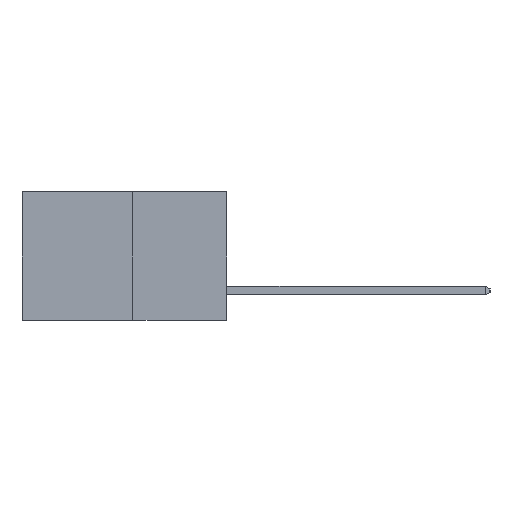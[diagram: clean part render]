
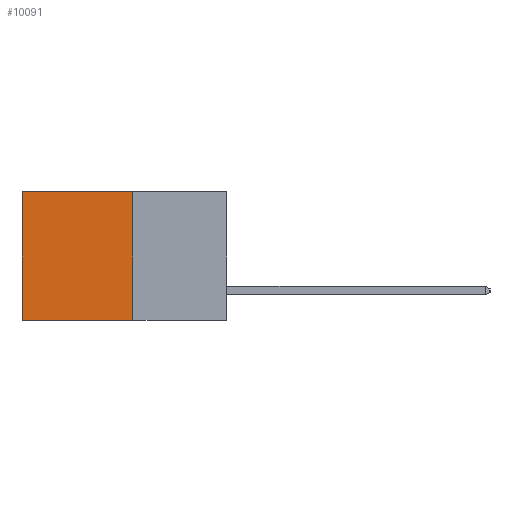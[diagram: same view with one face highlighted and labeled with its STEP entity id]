
A CAD part, left-side view. The second image highlights one B-rep face of the part: STEP entity #10091.
In plain terms, the highlighted planar face has unit normal (-1, 0, 0).
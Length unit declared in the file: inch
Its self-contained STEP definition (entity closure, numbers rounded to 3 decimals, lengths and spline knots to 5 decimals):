
#13 = VECTOR ( 'NONE', #5022, 39.37008 ) ;
#99 = ORIENTED_EDGE ( 'NONE', *, *, #27115, .F. ) ;
#935 = CARTESIAN_POINT ( 'NONE',  ( 0.277, 0.59, 0. ) ) ;
#1046 = VERTEX_POINT ( 'NONE', #8114 ) ;
#1175 = CARTESIAN_POINT ( 'NONE',  ( 0.277, 0.59, -0.37 ) ) ;
#1404 = VECTOR ( 'NONE', #1631, 39.37008 ) ;
#1631 = DIRECTION ( 'NONE',  ( 0., 1., 0. ) ) ;
#1687 = CARTESIAN_POINT ( 'NONE',  ( 0.277, 0.27, -0.37 ) ) ;
#2156 = LINE ( 'NONE', #15811, #1404 ) ;
#2354 = ORIENTED_EDGE ( 'NONE', *, *, #24968, .T. ) ;
#2947 = FACE_OUTER_BOUND ( 'NONE', #23746, .T. ) ;
#3757 = CARTESIAN_POINT ( 'NONE',  ( 0.277, 0.59, -0.37 ) ) ;
#5022 = DIRECTION ( 'NONE',  ( 0., 1., 0. ) ) ;
#5346 = VERTEX_POINT ( 'NONE', #1175 ) ;
#6203 = CARTESIAN_POINT ( 'NONE',  ( 0.277, 0.27, -0.37 ) ) ;
#6431 = LINE ( 'NONE', #12138, #13 ) ;
#8114 = CARTESIAN_POINT ( 'NONE',  ( 0.277, 0.27, 0. ) ) ;
#8380 = VERTEX_POINT ( 'NONE', #935 ) ;
#8600 = DIRECTION ( 'NONE',  ( 0., 0., -1. ) ) ;
#10091 = ADVANCED_FACE ( 'NONE', ( #2947 ), #17966, .F. ) ;
#12138 = CARTESIAN_POINT ( 'NONE',  ( 0.277, 0.27, -0.37 ) ) ;
#13581 = ORIENTED_EDGE ( 'NONE', *, *, #28150, .F. ) ;
#15106 = VECTOR ( 'NONE', #24900, 39.37008 ) ;
#15811 = CARTESIAN_POINT ( 'NONE',  ( 0.277, 0.27, 0. ) ) ;
#17966 = PLANE ( 'NONE',  #28565 ) ;
#18531 = VECTOR ( 'NONE', #20636, 39.37008 ) ;
#19149 = EDGE_CURVE ( 'NONE', #8380, #5346, #21257, .T. ) ;
#20636 = DIRECTION ( 'NONE',  ( 0., 0., -1. ) ) ;
#21257 = LINE ( 'NONE', #3757, #15106 ) ;
#22591 = DIRECTION ( 'NONE',  ( 1., 0., 0. ) ) ;
#23746 = EDGE_LOOP ( 'NONE', ( #27624, #99, #13581, #2354 ) ) ;
#24362 = CARTESIAN_POINT ( 'NONE',  ( 0.277, 0.27, -0.37 ) ) ;
#24620 = LINE ( 'NONE', #1687, #18531 ) ;
#24786 = VERTEX_POINT ( 'NONE', #24362 ) ;
#24900 = DIRECTION ( 'NONE',  ( 0., 0., -1. ) ) ;
#24968 = EDGE_CURVE ( 'NONE', #1046, #8380, #2156, .T. ) ;
#27115 = EDGE_CURVE ( 'NONE', #24786, #5346, #6431, .T. ) ;
#27624 = ORIENTED_EDGE ( 'NONE', *, *, #19149, .T. ) ;
#28150 = EDGE_CURVE ( 'NONE', #1046, #24786, #24620, .T. ) ;
#28565 = AXIS2_PLACEMENT_3D ( 'NONE', #6203, #22591, #8600 ) ;
